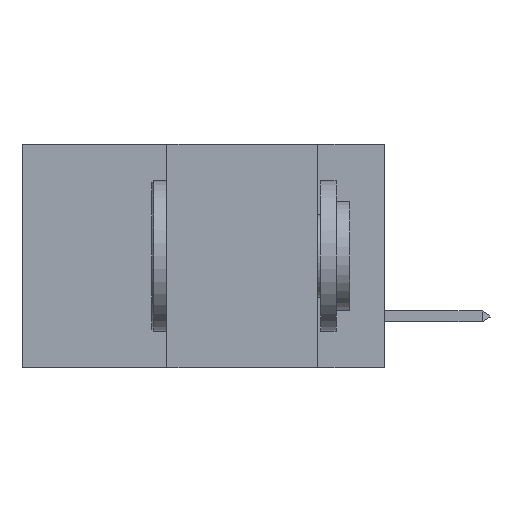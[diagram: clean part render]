
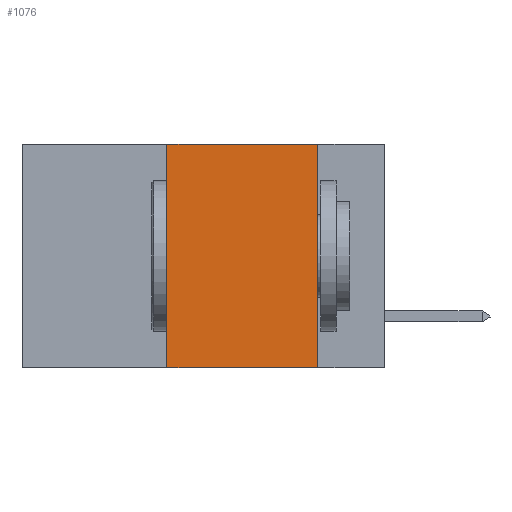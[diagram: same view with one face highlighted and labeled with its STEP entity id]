
A CAD part, left-side view. The second image highlights one B-rep face of the part: STEP entity #1076.
In plain terms, the highlighted planar face has unit normal (-1, 0, 0).
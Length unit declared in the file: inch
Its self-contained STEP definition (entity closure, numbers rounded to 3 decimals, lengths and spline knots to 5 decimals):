
#477 = DIRECTION ( 'NONE',  ( 0., 0., 1. ) ) ;
#767 = CARTESIAN_POINT ( 'NONE',  ( 0., 0.36, -0.37 ) ) ;
#1076 = ADVANCED_FACE ( 'NONE', ( #5733 ), #2460, .F. ) ;
#1129 = CARTESIAN_POINT ( 'NONE',  ( 0., 0.11, -0.37 ) ) ;
#2460 = PLANE ( 'NONE',  #17166 ) ;
#2695 = CARTESIAN_POINT ( 'NONE',  ( 0., 0.6, 0. ) ) ;
#3560 = ORIENTED_EDGE ( 'NONE', *, *, #13038, .F. ) ;
#4269 = CARTESIAN_POINT ( 'NONE',  ( 0., 0.36, 0. ) ) ;
#4336 = CARTESIAN_POINT ( 'NONE',  ( 0., 0.36, 0. ) ) ;
#5683 = EDGE_CURVE ( 'NONE', #21219, #15350, #23654, .T. ) ;
#5733 = FACE_OUTER_BOUND ( 'NONE', #10279, .T. ) ;
#6061 = DIRECTION ( 'NONE',  ( 0., 0., -1. ) ) ;
#6564 = DIRECTION ( 'NONE',  ( 0., -1., 0. ) ) ;
#6737 = VECTOR ( 'NONE', #6564, 39.37008 ) ;
#7218 = VERTEX_POINT ( 'NONE', #767 ) ;
#8125 = CARTESIAN_POINT ( 'NONE',  ( 0., 0.6, 0. ) ) ;
#8465 = CARTESIAN_POINT ( 'NONE',  ( 0., 0.11, 0. ) ) ;
#9416 = EDGE_CURVE ( 'NONE', #7218, #15350, #24489, .T. ) ;
#10279 = EDGE_LOOP ( 'NONE', ( #18829, #21728, #3560, #22653 ) ) ;
#13038 = EDGE_CURVE ( 'NONE', #7218, #16984, #15103, .T. ) ;
#14478 = VECTOR ( 'NONE', #477, 39.37008 ) ;
#14976 = DIRECTION ( 'NONE',  ( 0., 0., -1. ) ) ;
#15103 = LINE ( 'NONE', #4269, #14478 ) ;
#15350 = VERTEX_POINT ( 'NONE', #1129 ) ;
#15677 = VECTOR ( 'NONE', #23428, 39.37008 ) ;
#16784 = EDGE_CURVE ( 'NONE', #16984, #21219, #24949, .T. ) ;
#16984 = VERTEX_POINT ( 'NONE', #4336 ) ;
#17166 = AXIS2_PLACEMENT_3D ( 'NONE', #8125, #21682, #6061 ) ;
#18829 = ORIENTED_EDGE ( 'NONE', *, *, #5683, .F. ) ;
#19022 = CARTESIAN_POINT ( 'NONE',  ( 0., 0.6, -0.37 ) ) ;
#19097 = VECTOR ( 'NONE', #14976, 39.37008 ) ;
#21219 = VERTEX_POINT ( 'NONE', #8465 ) ;
#21682 = DIRECTION ( 'NONE',  ( 1., 0., 0. ) ) ;
#21728 = ORIENTED_EDGE ( 'NONE', *, *, #16784, .F. ) ;
#22653 = ORIENTED_EDGE ( 'NONE', *, *, #9416, .T. ) ;
#23428 = DIRECTION ( 'NONE',  ( 0., -1., 0. ) ) ;
#23654 = LINE ( 'NONE', #24742, #19097 ) ;
#24489 = LINE ( 'NONE', #19022, #15677 ) ;
#24742 = CARTESIAN_POINT ( 'NONE',  ( 0., 0.11, 0. ) ) ;
#24949 = LINE ( 'NONE', #2695, #6737 ) ;
